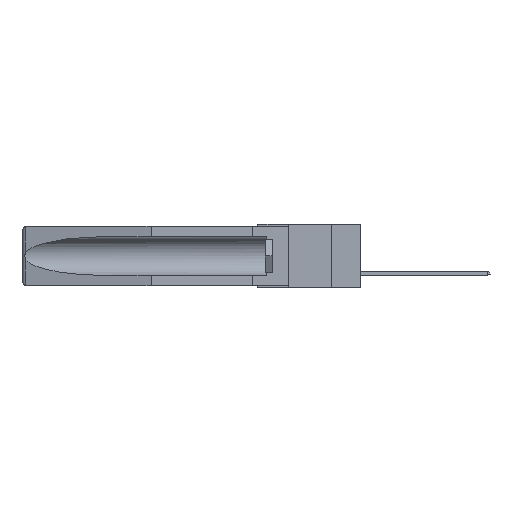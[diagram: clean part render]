
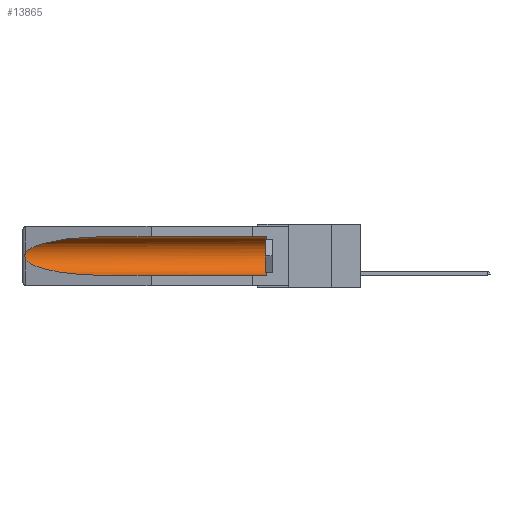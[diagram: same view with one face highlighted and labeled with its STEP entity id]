
A CAD part, left-side view. The second image highlights one B-rep face of the part: STEP entity #13865.
In plain terms, the highlighted cylindrical face has radius 2.857 mm (diameter 5.715 mm), a partial arc.
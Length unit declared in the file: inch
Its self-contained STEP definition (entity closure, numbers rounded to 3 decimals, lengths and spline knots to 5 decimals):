
#70 = ORIENTED_EDGE ( 'NONE', *, *, #14423, .T. ) ;
#824 = CARTESIAN_POINT ( 'NONE',  ( 0.155, 0.126, -0.059 ) ) ;
#1093 = CARTESIAN_POINT ( 'NONE',  ( 0.21114, 1.30732, -0.059 ) ) ;
#1097 = AXIS2_PLACEMENT_3D ( 'NONE', #12916, #15865, #13058 ) ;
#1159 = CARTESIAN_POINT ( 'NONE',  ( 0.21114, 1.30732, -0.284 ) ) ;
#1513 = DIRECTION ( 'NONE',  ( 0., 0., 1. ) ) ;
#1627 =( BOUNDED_CURVE ( )  B_SPLINE_CURVE ( 3, ( #8823, #1093, #11787, #14735 ),
 .UNSPECIFIED., .F., .F. ) 
 B_SPLINE_CURVE_WITH_KNOTS ( ( 4, 4 ),
 ( 4.71239, 6.08839 ),
 .UNSPECIFIED. ) 
 CURVE ( )  GEOMETRIC_REPRESENTATION_ITEM ( )  RATIONAL_B_SPLINE_CURVE ( ( 1., 0.848, 0.848, 1. ) ) 
 REPRESENTATION_ITEM ( '' )  );
#1642 = DIRECTION ( 'NONE',  ( 0., -1., 0. ) ) ;
#2353 = CARTESIAN_POINT ( 'NONE',  ( 0.155, -0.30754, -0.059 ) ) ;
#2901 = ORIENTED_EDGE ( 'NONE', *, *, #12928, .T. ) ;
#2907 = LINE ( 'NONE', #3128, #16076 ) ;
#2957 = EDGE_CURVE ( 'NONE', #14670, #9667, #1627, .T. ) ;
#3128 = CARTESIAN_POINT ( 'NONE',  ( 0.155, -0.30754, -0.284 ) ) ;
#3667 =( BOUNDED_CURVE ( )  B_SPLINE_CURVE ( 3, ( #5557, #16106, #1159, #17687 ),
 .UNSPECIFIED., .F., .F. ) 
 B_SPLINE_CURVE_WITH_KNOTS ( ( 4, 4 ),
 ( 0.1948, 1.5708 ),
 .UNSPECIFIED. ) 
 CURVE ( )  GEOMETRIC_REPRESENTATION_ITEM ( )  RATIONAL_B_SPLINE_CURVE ( ( 1., 0.848, 0.848, 1. ) ) 
 REPRESENTATION_ITEM ( '' )  );
#4345 = CARTESIAN_POINT ( 'NONE',  ( 0.155, 0.126, -0.284 ) ) ;
#4706 = CARTESIAN_POINT ( 'NONE',  ( 0.2673, 1.53269, -0.17917 ) ) ;
#4773 = CARTESIAN_POINT ( 'NONE',  ( 0.2673, 1.5327, -0.16383 ) ) ;
#5354 = DIRECTION ( 'NONE',  ( 0., 1., 0. ) ) ;
#5474 = CARTESIAN_POINT ( 'NONE',  ( 0.26537, 1.52718, -0.19328 ) ) ;
#5557 = CARTESIAN_POINT ( 'NONE',  ( 0.26537, 1.52718, -0.19328 ) ) ;
#5899 = ORIENTED_EDGE ( 'NONE', *, *, #2957, .T. ) ;
#6084 = AXIS2_PLACEMENT_3D ( 'NONE', #9038, #1642, #1513 ) ;
#6203 = CARTESIAN_POINT ( 'NONE',  ( 0.2675, 1.53308, -0.16763 ) ) ;
#6463 = CARTESIAN_POINT ( 'NONE',  ( 0.26597, 1.52961, -0.15275 ) ) ;
#7084 = VERTEX_POINT ( 'NONE', #4345 ) ;
#7181 = B_SPLINE_CURVE_WITH_KNOTS ( 'NONE', 3,
 ( #18435, #6463, #13814, #4773, #6203, #18493, #4706, #18300, #9451, #10850 ),
 .UNSPECIFIED., .F., .F.,
 ( 4, 2, 2, 2, 4 ),
 ( 0., 0.00029, 0.00058, 0.00087, 0.00117 ),
 .UNSPECIFIED. ) ;
#8347 = LINE ( 'NONE', #2353, #16348 ) ;
#8649 = EDGE_CURVE ( 'NONE', #7084, #13402, #16446, .T. ) ;
#8823 = CARTESIAN_POINT ( 'NONE',  ( 0.155, 1.07973, -0.059 ) ) ;
#8859 = ORIENTED_EDGE ( 'NONE', *, *, #8649, .T. ) ;
#9038 = CARTESIAN_POINT ( 'NONE',  ( 0.155, 0.126, -0.1715 ) ) ;
#9451 = CARTESIAN_POINT ( 'NONE',  ( 0.26597, 1.5296, -0.19026 ) ) ;
#9667 = VERTEX_POINT ( 'NONE', #17407 ) ;
#10292 = EDGE_CURVE ( 'NONE', #7084, #11802, #2907, .T. ) ;
#10610 = CARTESIAN_POINT ( 'NONE',  ( 0.155, 1.07973, -0.059 ) ) ;
#10766 = DIRECTION ( 'NONE',  ( 0., 1., 0. ) ) ;
#10850 = CARTESIAN_POINT ( 'NONE',  ( 0.26537, 1.52718, -0.19328 ) ) ;
#11787 = CARTESIAN_POINT ( 'NONE',  ( 0.25451, 1.48313, -0.09465 ) ) ;
#11802 = VERTEX_POINT ( 'NONE', #14912 ) ;
#12146 = FACE_OUTER_BOUND ( 'NONE', #15930, .T. ) ;
#12807 = ORIENTED_EDGE ( 'NONE', *, *, #10292, .F. ) ;
#12916 = CARTESIAN_POINT ( 'NONE',  ( 0.155, -0.30754, -0.1715 ) ) ;
#12928 = EDGE_CURVE ( 'NONE', #9667, #16184, #7181, .T. ) ;
#13058 = DIRECTION ( 'NONE',  ( 0., 0., 1. ) ) ;
#13402 = VERTEX_POINT ( 'NONE', #824 ) ;
#13572 = CYLINDRICAL_SURFACE ( 'NONE', #1097, 0.1125 ) ;
#13814 = CARTESIAN_POINT ( 'NONE',  ( 0.26654, 1.53092, -0.15636 ) ) ;
#13865 = ADVANCED_FACE ( 'NONE', ( #12146 ), #13572, .F. ) ;
#14423 = EDGE_CURVE ( 'NONE', #13402, #14670, #8347, .T. ) ;
#14670 = VERTEX_POINT ( 'NONE', #10610 ) ;
#14735 = CARTESIAN_POINT ( 'NONE',  ( 0.26537, 1.52718, -0.14972 ) ) ;
#14912 = CARTESIAN_POINT ( 'NONE',  ( 0.155, 1.07973, -0.284 ) ) ;
#15840 = ORIENTED_EDGE ( 'NONE', *, *, #16894, .T. ) ;
#15865 = DIRECTION ( 'NONE',  ( 0., 1., 0. ) ) ;
#15930 = EDGE_LOOP ( 'NONE', ( #5899, #2901, #15840, #12807, #8859, #70 ) ) ;
#16076 = VECTOR ( 'NONE', #10766, 39.37008 ) ;
#16106 = CARTESIAN_POINT ( 'NONE',  ( 0.25451, 1.48313, -0.24835 ) ) ;
#16184 = VERTEX_POINT ( 'NONE', #5474 ) ;
#16348 = VECTOR ( 'NONE', #5354, 39.37008 ) ;
#16446 = CIRCLE ( 'NONE', #6084, 0.1125 ) ;
#16894 = EDGE_CURVE ( 'NONE', #16184, #11802, #3667, .T. ) ;
#17407 = CARTESIAN_POINT ( 'NONE',  ( 0.26537, 1.52718, -0.14972 ) ) ;
#17687 = CARTESIAN_POINT ( 'NONE',  ( 0.155, 1.07973, -0.284 ) ) ;
#18300 = CARTESIAN_POINT ( 'NONE',  ( 0.26655, 1.53094, -0.18657 ) ) ;
#18435 = CARTESIAN_POINT ( 'NONE',  ( 0.26537, 1.52718, -0.14972 ) ) ;
#18493 = CARTESIAN_POINT ( 'NONE',  ( 0.2675, 1.53308, -0.17534 ) ) ;
